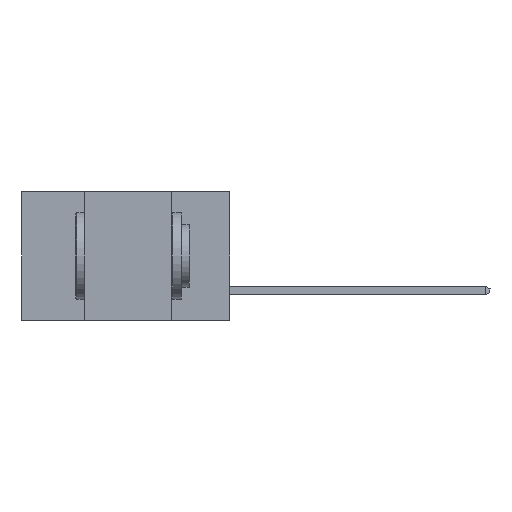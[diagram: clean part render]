
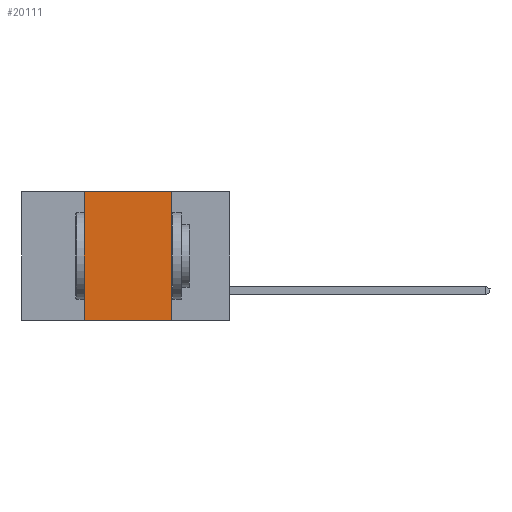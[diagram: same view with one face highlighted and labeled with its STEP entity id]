
A CAD part, left-side view. The second image highlights one B-rep face of the part: STEP entity #20111.
In plain terms, the highlighted planar face has unit normal (-1, 0, 0).
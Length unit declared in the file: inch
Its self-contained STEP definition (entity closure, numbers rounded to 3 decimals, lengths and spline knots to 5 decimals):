
#1104 = PLANE ( 'NONE',  #7848 ) ;
#1446 = FACE_OUTER_BOUND ( 'NONE', #13416, .T. ) ;
#2024 = LINE ( 'NONE', #6954, #3769 ) ;
#2117 = CARTESIAN_POINT ( 'NONE',  ( 0., 0.42, -0.37 ) ) ;
#3769 = VECTOR ( 'NONE', #19168, 39.37008 ) ;
#4204 = CARTESIAN_POINT ( 'NONE',  ( 0., 0.42, 0. ) ) ;
#4588 = DIRECTION ( 'NONE',  ( 1., 0., 0. ) ) ;
#4601 = EDGE_CURVE ( 'NONE', #17841, #18283, #13764, .T. ) ;
#4731 = CARTESIAN_POINT ( 'NONE',  ( 0., 0.17, -0.37 ) ) ;
#5459 = VERTEX_POINT ( 'NONE', #12159 ) ;
#6247 = ORIENTED_EDGE ( 'NONE', *, *, #20306, .F. ) ;
#6642 = ORIENTED_EDGE ( 'NONE', *, *, #19096, .F. ) ;
#6954 = CARTESIAN_POINT ( 'NONE',  ( 0., 0.6, 0. ) ) ;
#7074 = VECTOR ( 'NONE', #12185, 39.37008 ) ;
#7848 = AXIS2_PLACEMENT_3D ( 'NONE', #10081, #4588, #11439 ) ;
#9663 = VECTOR ( 'NONE', #14725, 39.37008 ) ;
#9993 = ORIENTED_EDGE ( 'NONE', *, *, #4601, .T. ) ;
#10081 = CARTESIAN_POINT ( 'NONE',  ( 0., 0.6, 0. ) ) ;
#11182 = DIRECTION ( 'NONE',  ( 0., 0., 1. ) ) ;
#11439 = DIRECTION ( 'NONE',  ( 0., 0., -1. ) ) ;
#12159 = CARTESIAN_POINT ( 'NONE',  ( 0., 0.17, 0. ) ) ;
#12185 = DIRECTION ( 'NONE',  ( 0., -1., 0. ) ) ;
#13190 = ORIENTED_EDGE ( 'NONE', *, *, #14148, .F. ) ;
#13267 = LINE ( 'NONE', #4731, #9663 ) ;
#13416 = EDGE_LOOP ( 'NONE', ( #6642, #13190, #6247, #9993 ) ) ;
#13651 = CARTESIAN_POINT ( 'NONE',  ( 0., 0.17, -0.37 ) ) ;
#13657 = VERTEX_POINT ( 'NONE', #4204 ) ;
#13764 = LINE ( 'NONE', #20697, #7074 ) ;
#14148 = EDGE_CURVE ( 'NONE', #13657, #5459, #2024, .T. ) ;
#14291 = VECTOR ( 'NONE', #11182, 39.37008 ) ;
#14725 = DIRECTION ( 'NONE',  ( 0., 0., -1. ) ) ;
#17841 = VERTEX_POINT ( 'NONE', #2117 ) ;
#18283 = VERTEX_POINT ( 'NONE', #13651 ) ;
#19096 = EDGE_CURVE ( 'NONE', #5459, #18283, #13267, .T. ) ;
#19168 = DIRECTION ( 'NONE',  ( 0., -1., 0. ) ) ;
#19254 = LINE ( 'NONE', #19699, #14291 ) ;
#19699 = CARTESIAN_POINT ( 'NONE',  ( 0., 0.42, -0.37 ) ) ;
#20111 = ADVANCED_FACE ( 'NONE', ( #1446 ), #1104, .F. ) ;
#20306 = EDGE_CURVE ( 'NONE', #17841, #13657, #19254, .T. ) ;
#20697 = CARTESIAN_POINT ( 'NONE',  ( 0., 0.6, -0.37 ) ) ;
